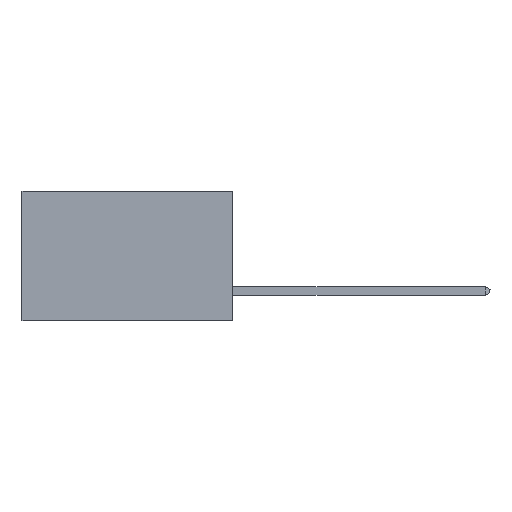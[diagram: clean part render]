
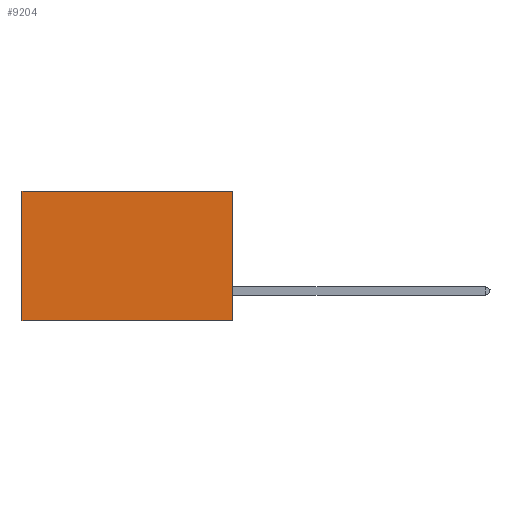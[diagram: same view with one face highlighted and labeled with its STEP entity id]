
A CAD part, left-side view. The second image highlights one B-rep face of the part: STEP entity #9204.
In plain terms, the highlighted planar face has unit normal (-1, 0, 0).
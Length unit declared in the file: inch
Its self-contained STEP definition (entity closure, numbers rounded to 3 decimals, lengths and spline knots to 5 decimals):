
#238 = ORIENTED_EDGE ( 'NONE', *, *, #23061, .F. ) ;
#2396 = VECTOR ( 'NONE', #33601, 39.37008 ) ;
#4104 = VERTEX_POINT ( 'NONE', #42018 ) ;
#4325 = EDGE_CURVE ( 'NONE', #42913, #43104, #11772, .T. ) ;
#6144 = DIRECTION ( 'NONE',  ( 1., 0., 0. ) ) ;
#8123 = ORIENTED_EDGE ( 'NONE', *, *, #26171, .T. ) ;
#9204 = ADVANCED_FACE ( 'NONE', ( #31015 ), #46834, .F. ) ;
#11772 = LINE ( 'NONE', #20184, #15387 ) ;
#12905 = CARTESIAN_POINT ( 'NONE',  ( 0.2875, 0.6, 0. ) ) ;
#13716 = CARTESIAN_POINT ( 'NONE',  ( 0.2875, 0.6, 0. ) ) ;
#14486 = CARTESIAN_POINT ( 'NONE',  ( 0.2875, 0., -0.37 ) ) ;
#15387 = VECTOR ( 'NONE', #36634, 39.37008 ) ;
#18210 = CARTESIAN_POINT ( 'NONE',  ( 0.2875, 0.6, -0.37 ) ) ;
#18872 = VERTEX_POINT ( 'NONE', #18210 ) ;
#20184 = CARTESIAN_POINT ( 'NONE',  ( 0.2875, 0., 0. ) ) ;
#21361 = EDGE_LOOP ( 'NONE', ( #8123, #238, #22735, #47483 ) ) ;
#22735 = ORIENTED_EDGE ( 'NONE', *, *, #31755, .F. ) ;
#23061 = EDGE_CURVE ( 'NONE', #4104, #18872, #46968, .T. ) ;
#24278 = VECTOR ( 'NONE', #32568, 39.37008 ) ;
#26171 = EDGE_CURVE ( 'NONE', #43104, #18872, #36292, .T. ) ;
#26280 = VECTOR ( 'NONE', #39229, 39.37008 ) ;
#31015 = FACE_OUTER_BOUND ( 'NONE', #21361, .T. ) ;
#31755 = EDGE_CURVE ( 'NONE', #42913, #4104, #45832, .T. ) ;
#32018 = AXIS2_PLACEMENT_3D ( 'NONE', #39367, #6144, #32772 ) ;
#32568 = DIRECTION ( 'NONE',  ( 0., 0., -1. ) ) ;
#32772 = DIRECTION ( 'NONE',  ( 0., 0., -1. ) ) ;
#33601 = DIRECTION ( 'NONE',  ( 0., 1., 0. ) ) ;
#36292 = LINE ( 'NONE', #12905, #26280 ) ;
#36634 = DIRECTION ( 'NONE',  ( 0., 1., 0. ) ) ;
#36955 = CARTESIAN_POINT ( 'NONE',  ( 0.2875, 0., 0. ) ) ;
#39229 = DIRECTION ( 'NONE',  ( 0., 0., -1. ) ) ;
#39367 = CARTESIAN_POINT ( 'NONE',  ( 0.2875, 0., 0. ) ) ;
#42018 = CARTESIAN_POINT ( 'NONE',  ( 0.2875, 0., -0.37 ) ) ;
#42913 = VERTEX_POINT ( 'NONE', #48655 ) ;
#43104 = VERTEX_POINT ( 'NONE', #13716 ) ;
#45832 = LINE ( 'NONE', #36955, #24278 ) ;
#46834 = PLANE ( 'NONE',  #32018 ) ;
#46968 = LINE ( 'NONE', #14486, #2396 ) ;
#47483 = ORIENTED_EDGE ( 'NONE', *, *, #4325, .T. ) ;
#48655 = CARTESIAN_POINT ( 'NONE',  ( 0.2875, 0., 0. ) ) ;
